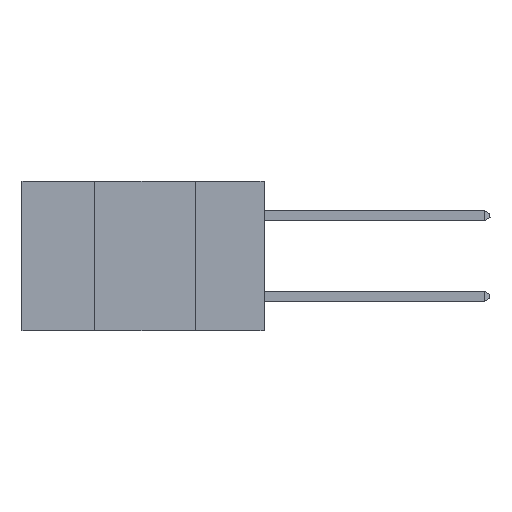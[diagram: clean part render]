
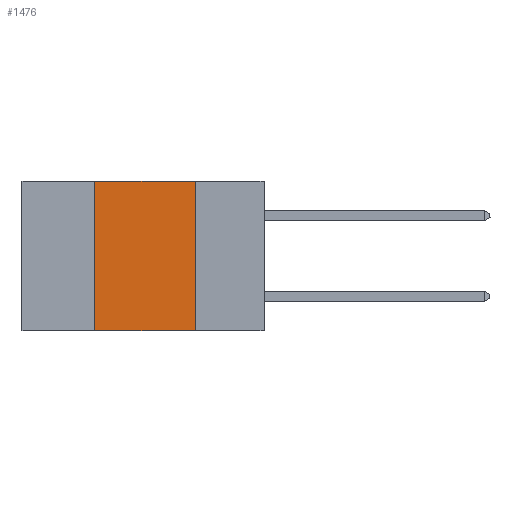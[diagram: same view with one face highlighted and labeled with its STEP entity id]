
A CAD part, left-side view. The second image highlights one B-rep face of the part: STEP entity #1476.
In plain terms, the highlighted planar face has unit normal (-1, 0, 0).
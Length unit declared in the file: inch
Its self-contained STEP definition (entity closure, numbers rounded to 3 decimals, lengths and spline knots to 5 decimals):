
#991 = LINE ( 'NONE', #5184, #4399 ) ;
#1031 = LINE ( 'NONE', #9277, #8557 ) ;
#1056 = LINE ( 'NONE', #7382, #2080 ) ;
#1253 = DIRECTION ( 'NONE',  ( 0., 0., -1. ) ) ;
#1476 = ADVANCED_FACE ( 'NONE', ( #4926 ), #7838, .F. ) ;
#1932 = ORIENTED_EDGE ( 'NONE', *, *, #3013, .F. ) ;
#2080 = VECTOR ( 'NONE', #9479, 39.37008 ) ;
#2747 = CARTESIAN_POINT ( 'NONE',  ( 0., 0.42, -0.37 ) ) ;
#2756 = CARTESIAN_POINT ( 'NONE',  ( 0., 0.17, -0.37 ) ) ;
#3010 = ORIENTED_EDGE ( 'NONE', *, *, #7717, .T. ) ;
#3013 = EDGE_CURVE ( 'NONE', #4707, #4182, #1056, .T. ) ;
#3388 = CARTESIAN_POINT ( 'NONE',  ( 0., 0.6, -0.37 ) ) ;
#3907 = CARTESIAN_POINT ( 'NONE',  ( 0., 0.17, 0. ) ) ;
#4182 = VERTEX_POINT ( 'NONE', #8886 ) ;
#4327 = EDGE_CURVE ( 'NONE', #6294, #7934, #1031, .T. ) ;
#4399 = VECTOR ( 'NONE', #4458, 39.37008 ) ;
#4458 = DIRECTION ( 'NONE',  ( 0., -1., 0. ) ) ;
#4707 = VERTEX_POINT ( 'NONE', #2747 ) ;
#4918 = DIRECTION ( 'NONE',  ( 0., -1., 0. ) ) ;
#4926 = FACE_OUTER_BOUND ( 'NONE', #5662, .T. ) ;
#5184 = CARTESIAN_POINT ( 'NONE',  ( 0., 0.6, 0. ) ) ;
#5662 = EDGE_LOOP ( 'NONE', ( #7917, #9080, #1932, #3010 ) ) ;
#6294 = VERTEX_POINT ( 'NONE', #3907 ) ;
#6461 = DIRECTION ( 'NONE',  ( 0., 0., -1. ) ) ;
#6763 = EDGE_CURVE ( 'NONE', #4182, #6294, #991, .T. ) ;
#7225 = DIRECTION ( 'NONE',  ( 1., 0., 0. ) ) ;
#7382 = CARTESIAN_POINT ( 'NONE',  ( 0., 0.42, 0. ) ) ;
#7717 = EDGE_CURVE ( 'NONE', #4707, #7934, #9201, .T. ) ;
#7838 = PLANE ( 'NONE',  #8632 ) ;
#7870 = CARTESIAN_POINT ( 'NONE',  ( 0., 0.6, 0. ) ) ;
#7917 = ORIENTED_EDGE ( 'NONE', *, *, #4327, .F. ) ;
#7934 = VERTEX_POINT ( 'NONE', #2756 ) ;
#8557 = VECTOR ( 'NONE', #1253, 39.37008 ) ;
#8632 = AXIS2_PLACEMENT_3D ( 'NONE', #7870, #7225, #6461 ) ;
#8886 = CARTESIAN_POINT ( 'NONE',  ( 0., 0.42, 0. ) ) ;
#9080 = ORIENTED_EDGE ( 'NONE', *, *, #6763, .F. ) ;
#9201 = LINE ( 'NONE', #3388, #9432 ) ;
#9277 = CARTESIAN_POINT ( 'NONE',  ( 0., 0.17, 0. ) ) ;
#9432 = VECTOR ( 'NONE', #4918, 39.37008 ) ;
#9479 = DIRECTION ( 'NONE',  ( 0., 0., 1. ) ) ;
